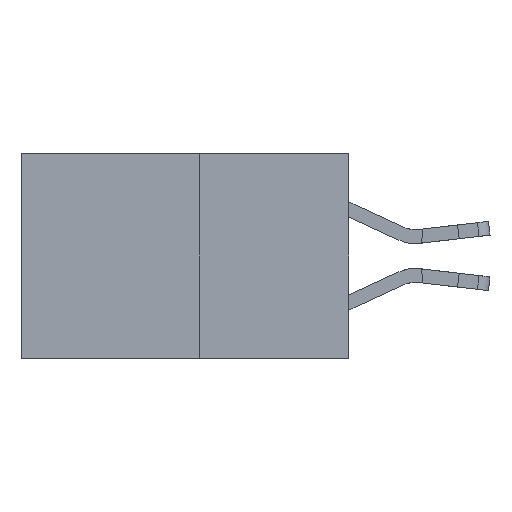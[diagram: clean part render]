
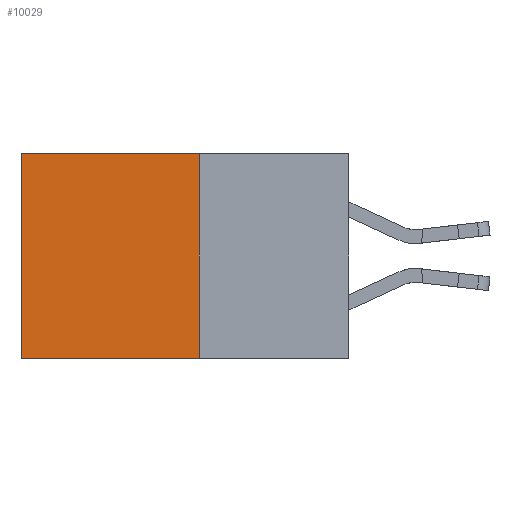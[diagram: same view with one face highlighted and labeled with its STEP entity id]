
A CAD part, left-side view. The second image highlights one B-rep face of the part: STEP entity #10029.
In plain terms, the highlighted planar face has unit normal (-1, 0, 0).
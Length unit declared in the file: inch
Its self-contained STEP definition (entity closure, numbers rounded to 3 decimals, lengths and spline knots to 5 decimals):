
#179 = DIRECTION ( 'NONE',  ( 0., 1., 0. ) ) ;
#338 = CARTESIAN_POINT ( 'NONE',  ( 0.277, 0.27, -0.37 ) ) ;
#616 = CARTESIAN_POINT ( 'NONE',  ( 0.277, 0.27, -0.37 ) ) ;
#880 = LINE ( 'NONE', #11256, #3907 ) ;
#938 = VERTEX_POINT ( 'NONE', #11475 ) ;
#991 = EDGE_CURVE ( 'NONE', #938, #12350, #3555, .T. ) ;
#2238 = LINE ( 'NONE', #338, #10908 ) ;
#2369 = CARTESIAN_POINT ( 'NONE',  ( 0.277, 0.59, 0. ) ) ;
#3406 = ORIENTED_EDGE ( 'NONE', *, *, #5828, .F. ) ;
#3555 = LINE ( 'NONE', #6475, #9274 ) ;
#3697 = AXIS2_PLACEMENT_3D ( 'NONE', #10941, #4194, #12025 ) ;
#3907 = VECTOR ( 'NONE', #10217, 39.37008 ) ;
#4062 = VECTOR ( 'NONE', #7819, 39.37008 ) ;
#4087 = EDGE_CURVE ( 'NONE', #938, #12846, #4426, .T. ) ;
#4194 = DIRECTION ( 'NONE',  ( 1., 0., 0. ) ) ;
#4426 = LINE ( 'NONE', #8016, #4062 ) ;
#4692 = ORIENTED_EDGE ( 'NONE', *, *, #991, .F. ) ;
#5828 = EDGE_CURVE ( 'NONE', #12350, #12371, #2238, .T. ) ;
#6475 = CARTESIAN_POINT ( 'NONE',  ( 0.277, 0.27, -0.37 ) ) ;
#7737 = ORIENTED_EDGE ( 'NONE', *, *, #4087, .T. ) ;
#7819 = DIRECTION ( 'NONE',  ( 0., 1., 0. ) ) ;
#8016 = CARTESIAN_POINT ( 'NONE',  ( 0.277, 0.27, 0. ) ) ;
#8793 = ORIENTED_EDGE ( 'NONE', *, *, #10824, .T. ) ;
#9274 = VECTOR ( 'NONE', #12991, 39.37008 ) ;
#10029 = ADVANCED_FACE ( 'NONE', ( #13989 ), #10898, .F. ) ;
#10217 = DIRECTION ( 'NONE',  ( 0., 0., -1. ) ) ;
#10824 = EDGE_CURVE ( 'NONE', #12846, #12371, #880, .T. ) ;
#10898 = PLANE ( 'NONE',  #3697 ) ;
#10908 = VECTOR ( 'NONE', #179, 39.37008 ) ;
#10941 = CARTESIAN_POINT ( 'NONE',  ( 0.277, 0.27, -0.37 ) ) ;
#11256 = CARTESIAN_POINT ( 'NONE',  ( 0.277, 0.59, -0.37 ) ) ;
#11475 = CARTESIAN_POINT ( 'NONE',  ( 0.277, 0.27, 0. ) ) ;
#11835 = CARTESIAN_POINT ( 'NONE',  ( 0.277, 0.59, -0.37 ) ) ;
#12025 = DIRECTION ( 'NONE',  ( 0., 0., -1. ) ) ;
#12350 = VERTEX_POINT ( 'NONE', #616 ) ;
#12371 = VERTEX_POINT ( 'NONE', #11835 ) ;
#12846 = VERTEX_POINT ( 'NONE', #2369 ) ;
#12991 = DIRECTION ( 'NONE',  ( 0., 0., -1. ) ) ;
#13989 = FACE_OUTER_BOUND ( 'NONE', #14260, .T. ) ;
#14260 = EDGE_LOOP ( 'NONE', ( #8793, #3406, #4692, #7737 ) ) ;
